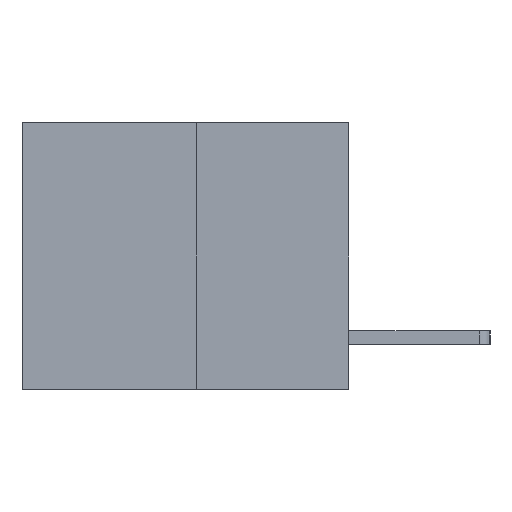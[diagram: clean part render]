
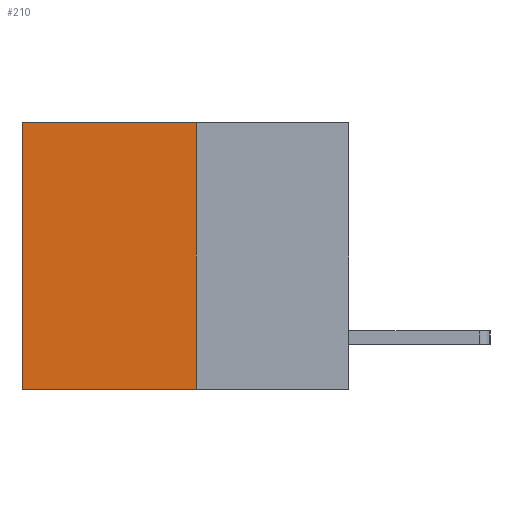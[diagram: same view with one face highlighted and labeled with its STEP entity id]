
A CAD part, left-side view. The second image highlights one B-rep face of the part: STEP entity #210.
In plain terms, the highlighted planar face has unit normal (-1, 0, 0).
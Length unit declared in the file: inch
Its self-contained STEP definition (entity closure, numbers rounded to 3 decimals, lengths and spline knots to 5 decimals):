
#210 = ADVANCED_FACE ( 'NONE', ( #6503 ), #7448, .F. ) ;
#404 = CARTESIAN_POINT ( 'NONE',  ( 0.3165, 0.28, 0. ) ) ;
#473 = CARTESIAN_POINT ( 'NONE',  ( 0.3165, 0.6, -0.49 ) ) ;
#863 = VECTOR ( 'NONE', #4180, 39.37008 ) ;
#1186 = CARTESIAN_POINT ( 'NONE',  ( 0.3165, 0.28, -0.49 ) ) ;
#1359 = ORIENTED_EDGE ( 'NONE', *, *, #7400, .T. ) ;
#1383 = EDGE_CURVE ( 'NONE', #3113, #6155, #4837, .T. ) ;
#1696 = DIRECTION ( 'NONE',  ( 0., 0., -1. ) ) ;
#1780 = VECTOR ( 'NONE', #8541, 39.37008 ) ;
#2140 = LINE ( 'NONE', #5971, #7552 ) ;
#2248 = EDGE_CURVE ( 'NONE', #3472, #4762, #2140, .T. ) ;
#3113 = VERTEX_POINT ( 'NONE', #404 ) ;
#3275 = ORIENTED_EDGE ( 'NONE', *, *, #1383, .T. ) ;
#3472 = VERTEX_POINT ( 'NONE', #6322 ) ;
#3656 = EDGE_CURVE ( 'NONE', #3113, #3472, #5661, .T. ) ;
#4180 = DIRECTION ( 'NONE',  ( 0., 1., 0. ) ) ;
#4762 = VERTEX_POINT ( 'NONE', #473 ) ;
#4837 = LINE ( 'NONE', #7893, #863 ) ;
#5183 = DIRECTION ( 'NONE',  ( 1., 0., 0. ) ) ;
#5255 = CARTESIAN_POINT ( 'NONE',  ( 0.3165, 0.6, 0. ) ) ;
#5479 = ORIENTED_EDGE ( 'NONE', *, *, #2248, .F. ) ;
#5661 = LINE ( 'NONE', #1186, #1780 ) ;
#5971 = CARTESIAN_POINT ( 'NONE',  ( 0.3165, 0.28, -0.49 ) ) ;
#6155 = VERTEX_POINT ( 'NONE', #5255 ) ;
#6174 = LINE ( 'NONE', #6995, #7941 ) ;
#6322 = CARTESIAN_POINT ( 'NONE',  ( 0.3165, 0.28, -0.49 ) ) ;
#6503 = FACE_OUTER_BOUND ( 'NONE', #9123, .T. ) ;
#6646 = CARTESIAN_POINT ( 'NONE',  ( 0.3165, 0.28, -0.49 ) ) ;
#6995 = CARTESIAN_POINT ( 'NONE',  ( 0.3165, 0.6, -0.49 ) ) ;
#7044 = AXIS2_PLACEMENT_3D ( 'NONE', #6646, #5183, #9663 ) ;
#7395 = DIRECTION ( 'NONE',  ( 0., 1., 0. ) ) ;
#7400 = EDGE_CURVE ( 'NONE', #6155, #4762, #6174, .T. ) ;
#7448 = PLANE ( 'NONE',  #7044 ) ;
#7552 = VECTOR ( 'NONE', #7395, 39.37008 ) ;
#7784 = ORIENTED_EDGE ( 'NONE', *, *, #3656, .F. ) ;
#7893 = CARTESIAN_POINT ( 'NONE',  ( 0.3165, 0.28, 0. ) ) ;
#7941 = VECTOR ( 'NONE', #1696, 39.37008 ) ;
#8541 = DIRECTION ( 'NONE',  ( 0., 0., -1. ) ) ;
#9123 = EDGE_LOOP ( 'NONE', ( #1359, #5479, #7784, #3275 ) ) ;
#9663 = DIRECTION ( 'NONE',  ( 0., 0., -1. ) ) ;
